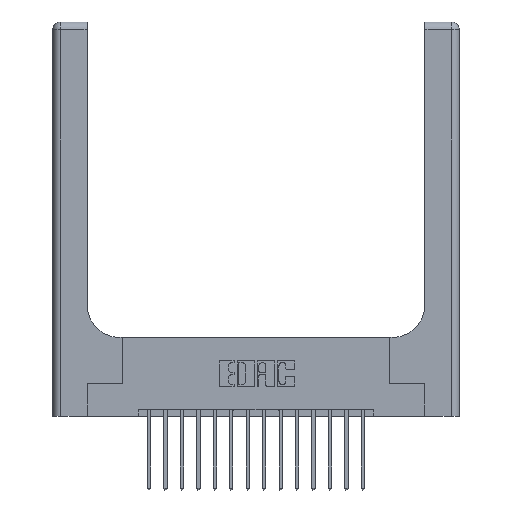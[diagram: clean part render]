
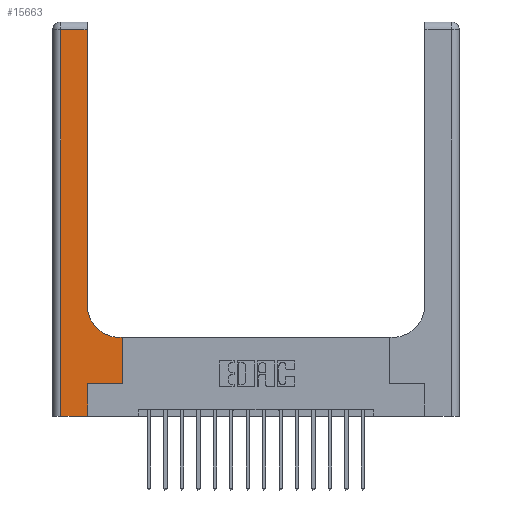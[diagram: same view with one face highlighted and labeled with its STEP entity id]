
A CAD part, top view. The second image highlights one B-rep face of the part: STEP entity #15663.
In plain terms, the highlighted planar face has unit normal (0, 0, 1).
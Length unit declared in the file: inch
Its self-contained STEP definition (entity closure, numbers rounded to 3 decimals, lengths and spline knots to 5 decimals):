
#336 = VECTOR ( 'NONE', #16576, 39.37008 ) ;
#1119 = EDGE_CURVE ( 'NONE', #8570, #2722, #10523, .T. ) ;
#1150 = ORIENTED_EDGE ( 'NONE', *, *, #18400, .T. ) ;
#1412 = CIRCLE ( 'NONE', #11913, 0.25 ) ;
#2130 = ORIENTED_EDGE ( 'NONE', *, *, #7274, .T. ) ;
#2276 = ORIENTED_EDGE ( 'NONE', *, *, #15731, .T. ) ;
#2671 = VECTOR ( 'NONE', #4907, 39.37008 ) ;
#2722 = VERTEX_POINT ( 'NONE', #5762 ) ;
#3036 = DIRECTION ( 'NONE',  ( 0., -1., 0. ) ) ;
#3240 = VERTEX_POINT ( 'NONE', #15470 ) ;
#3264 = DIRECTION ( 'NONE',  ( 1., 0., 0. ) ) ;
#3459 = LINE ( 'NONE', #8539, #4222 ) ;
#3478 = CARTESIAN_POINT ( 'NONE',  ( 0.265, 0.25, 0.37 ) ) ;
#3808 = EDGE_CURVE ( 'NONE', #17622, #9136, #18134, .T. ) ;
#3911 = CARTESIAN_POINT ( 'NONE',  ( 0.528, 0.25, 0.37 ) ) ;
#4169 = DIRECTION ( 'NONE',  ( -1., 0., 0. ) ) ;
#4222 = VECTOR ( 'NONE', #15304, 39.37008 ) ;
#4387 = ORIENTED_EDGE ( 'NONE', *, *, #10582, .T. ) ;
#4454 = CARTESIAN_POINT ( 'NONE',  ( 0.06, 3., 0.37 ) ) ;
#4665 = VERTEX_POINT ( 'NONE', #14158 ) ;
#4766 = ORIENTED_EDGE ( 'NONE', *, *, #1119, .T. ) ;
#4907 = DIRECTION ( 'NONE',  ( 1., 0., 0. ) ) ;
#5543 = VECTOR ( 'NONE', #14810, 39.37008 ) ;
#5762 = CARTESIAN_POINT ( 'NONE',  ( 0.265, 0., 0.37 ) ) ;
#5942 = DIRECTION ( 'NONE',  ( 1., 0., 0. ) ) ;
#5961 = VERTEX_POINT ( 'NONE', #3911 ) ;
#6140 = LINE ( 'NONE', #3478, #2671 ) ;
#6389 = LINE ( 'NONE', #12246, #5543 ) ;
#6598 = ORIENTED_EDGE ( 'NONE', *, *, #9379, .T. ) ;
#6796 = LINE ( 'NONE', #15243, #12121 ) ;
#6920 = ORIENTED_EDGE ( 'NONE', *, *, #11224, .T. ) ;
#7274 = EDGE_CURVE ( 'NONE', #3240, #4665, #6389, .T. ) ;
#7778 = VERTEX_POINT ( 'NONE', #10432 ) ;
#8514 = LINE ( 'NONE', #4454, #10151 ) ;
#8539 = CARTESIAN_POINT ( 'NONE',  ( 0.528, 0.25, 0.37 ) ) ;
#8570 = VERTEX_POINT ( 'NONE', #14484 ) ;
#8673 = VERTEX_POINT ( 'NONE', #15237 ) ;
#9136 = VERTEX_POINT ( 'NONE', #17470 ) ;
#9379 = EDGE_CURVE ( 'NONE', #7778, #5961, #6140, .T. ) ;
#10151 = VECTOR ( 'NONE', #3036, 39.37008 ) ;
#10182 = CARTESIAN_POINT ( 'NONE',  ( 0.265, 0., 0.37 ) ) ;
#10301 = DIRECTION ( 'NONE',  ( 0., 0., -1. ) ) ;
#10432 = CARTESIAN_POINT ( 'NONE',  ( 0.265, 0.25, 0.37 ) ) ;
#10523 = LINE ( 'NONE', #16170, #13224 ) ;
#10582 = EDGE_CURVE ( 'NONE', #5961, #3240, #3459, .T. ) ;
#10868 = ORIENTED_EDGE ( 'NONE', *, *, #3808, .T. ) ;
#11224 = EDGE_CURVE ( 'NONE', #8673, #17622, #6796, .T. ) ;
#11677 = CARTESIAN_POINT ( 'NONE',  ( 0., 3., 0.37 ) ) ;
#11742 = DIRECTION ( 'NONE',  ( 0., 1., 0. ) ) ;
#11913 = AXIS2_PLACEMENT_3D ( 'NONE', #14835, #17561, #5942 ) ;
#12121 = VECTOR ( 'NONE', #15525, 39.37008 ) ;
#12246 = CARTESIAN_POINT ( 'NONE',  ( 0.26, 0.6, 0.37 ) ) ;
#12302 = CARTESIAN_POINT ( 'NONE',  ( 0., 2.94, 0.37 ) ) ;
#12823 = AXIS2_PLACEMENT_3D ( 'NONE', #11677, #10301, #4169 ) ;
#13052 = LINE ( 'NONE', #10182, #17055 ) ;
#13195 = CARTESIAN_POINT ( 'NONE',  ( 0.26, 2.94, 0.37 ) ) ;
#13224 = VECTOR ( 'NONE', #3264, 39.37008 ) ;
#13276 = EDGE_LOOP ( 'NONE', ( #6920, #10868, #18081, #4766, #1150, #6598, #4387, #2130, #2276 ) ) ;
#14158 = CARTESIAN_POINT ( 'NONE',  ( 0.51, 0.6, 0.37 ) ) ;
#14484 = CARTESIAN_POINT ( 'NONE',  ( 0.06, 0., 0.37 ) ) ;
#14810 = DIRECTION ( 'NONE',  ( -1., 0., 0. ) ) ;
#14835 = CARTESIAN_POINT ( 'NONE',  ( 0.51, 0.85, 0.37 ) ) ;
#15237 = CARTESIAN_POINT ( 'NONE',  ( 0.26, 0.85, 0.37 ) ) ;
#15243 = CARTESIAN_POINT ( 'NONE',  ( 0.26, 3., 0.37 ) ) ;
#15304 = DIRECTION ( 'NONE',  ( 0., 1., 0. ) ) ;
#15470 = CARTESIAN_POINT ( 'NONE',  ( 0.528, 0.6, 0.37 ) ) ;
#15510 = EDGE_CURVE ( 'NONE', #9136, #8570, #8514, .T. ) ;
#15525 = DIRECTION ( 'NONE',  ( 0., 1., 0. ) ) ;
#15648 = FACE_OUTER_BOUND ( 'NONE', #13276, .T. ) ;
#15663 = ADVANCED_FACE ( 'NONE', ( #15648 ), #17041, .F. ) ;
#15731 = EDGE_CURVE ( 'NONE', #4665, #8673, #1412, .T. ) ;
#16170 = CARTESIAN_POINT ( 'NONE',  ( 0., 0., 0.37 ) ) ;
#16576 = DIRECTION ( 'NONE',  ( -1., 0., 0. ) ) ;
#17041 = PLANE ( 'NONE',  #12823 ) ;
#17055 = VECTOR ( 'NONE', #11742, 39.37008 ) ;
#17470 = CARTESIAN_POINT ( 'NONE',  ( 0.06, 2.94, 0.37 ) ) ;
#17561 = DIRECTION ( 'NONE',  ( 0., 0., -1. ) ) ;
#17622 = VERTEX_POINT ( 'NONE', #13195 ) ;
#18081 = ORIENTED_EDGE ( 'NONE', *, *, #15510, .T. ) ;
#18134 = LINE ( 'NONE', #12302, #336 ) ;
#18400 = EDGE_CURVE ( 'NONE', #2722, #7778, #13052, .T. ) ;
